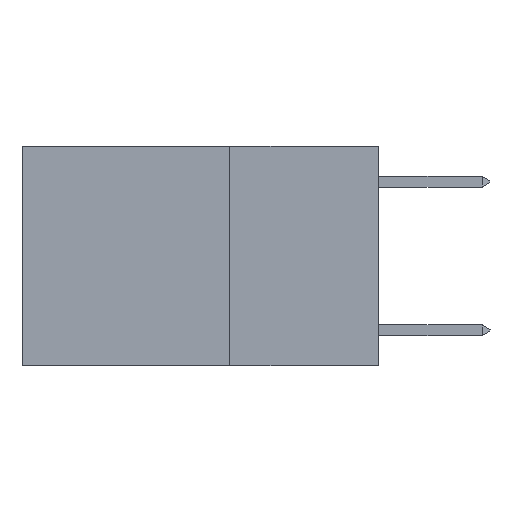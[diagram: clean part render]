
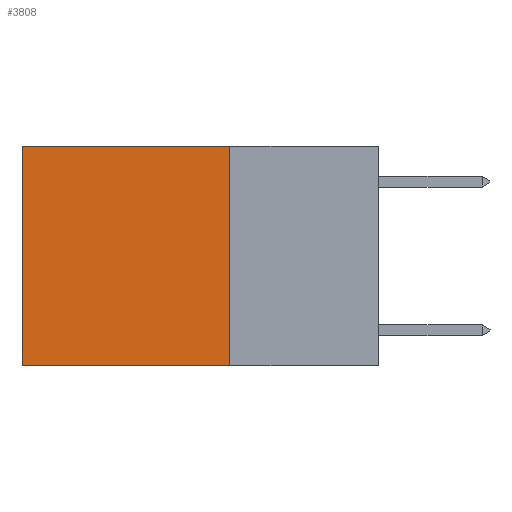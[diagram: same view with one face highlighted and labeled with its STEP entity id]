
A CAD part, left-side view. The second image highlights one B-rep face of the part: STEP entity #3808.
In plain terms, the highlighted planar face has unit normal (-1, 0, 0).
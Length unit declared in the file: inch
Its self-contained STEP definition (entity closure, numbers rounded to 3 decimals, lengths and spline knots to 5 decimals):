
#885 = CARTESIAN_POINT ( 'NONE',  ( 0.2625, 0.25, 0. ) ) ;
#1036 = VERTEX_POINT ( 'NONE', #885 ) ;
#1169 = CARTESIAN_POINT ( 'NONE',  ( 0.2625, 0.25, -0.37 ) ) ;
#1380 = DIRECTION ( 'NONE',  ( 0., 1., 0. ) ) ;
#1944 = VECTOR ( 'NONE', #23307, 39.37008 ) ;
#2574 = LINE ( 'NONE', #23353, #1944 ) ;
#2638 = EDGE_CURVE ( 'NONE', #3372, #15131, #9044, .T. ) ;
#2869 = EDGE_CURVE ( 'NONE', #1036, #23867, #6952, .T. ) ;
#3372 = VERTEX_POINT ( 'NONE', #23870 ) ;
#3589 = CARTESIAN_POINT ( 'NONE',  ( 0.2625, 0.6, -0.37 ) ) ;
#3808 = ADVANCED_FACE ( 'NONE', ( #20511 ), #8198, .F. ) ;
#4648 = ORIENTED_EDGE ( 'NONE', *, *, #2869, .F. ) ;
#4701 = ORIENTED_EDGE ( 'NONE', *, *, #2638, .T. ) ;
#6514 = VECTOR ( 'NONE', #7619, 39.37008 ) ;
#6952 = LINE ( 'NONE', #7565, #6514 ) ;
#7565 = CARTESIAN_POINT ( 'NONE',  ( 0.2625, 0.25, 0. ) ) ;
#7619 = DIRECTION ( 'NONE',  ( 0., 0., -1. ) ) ;
#7929 = DIRECTION ( 'NONE',  ( 0., 0., -1. ) ) ;
#7980 = DIRECTION ( 'NONE',  ( 1., 0., 0. ) ) ;
#8082 = CARTESIAN_POINT ( 'NONE',  ( 0.2625, 0.25, 0. ) ) ;
#8198 = PLANE ( 'NONE',  #23830 ) ;
#8759 = VECTOR ( 'NONE', #10515, 39.37008 ) ;
#8816 = ORIENTED_EDGE ( 'NONE', *, *, #11982, .F. ) ;
#9044 = LINE ( 'NONE', #10491, #8759 ) ;
#9880 = EDGE_CURVE ( 'NONE', #1036, #3372, #2574, .T. ) ;
#9975 = EDGE_LOOP ( 'NONE', ( #4701, #8816, #4648, #14585 ) ) ;
#10491 = CARTESIAN_POINT ( 'NONE',  ( 0.2625, 0.6, 0. ) ) ;
#10515 = DIRECTION ( 'NONE',  ( 0., 0., -1. ) ) ;
#11982 = EDGE_CURVE ( 'NONE', #23867, #15131, #12876, .T. ) ;
#12734 = VECTOR ( 'NONE', #1380, 39.37008 ) ;
#12876 = LINE ( 'NONE', #1169, #12734 ) ;
#14585 = ORIENTED_EDGE ( 'NONE', *, *, #9880, .T. ) ;
#15131 = VERTEX_POINT ( 'NONE', #3589 ) ;
#20511 = FACE_OUTER_BOUND ( 'NONE', #9975, .T. ) ;
#23307 = DIRECTION ( 'NONE',  ( 0., 1., 0. ) ) ;
#23353 = CARTESIAN_POINT ( 'NONE',  ( 0.2625, 0.25, 0. ) ) ;
#23707 = CARTESIAN_POINT ( 'NONE',  ( 0.2625, 0.25, -0.37 ) ) ;
#23830 = AXIS2_PLACEMENT_3D ( 'NONE', #8082, #7980, #7929 ) ;
#23867 = VERTEX_POINT ( 'NONE', #23707 ) ;
#23870 = CARTESIAN_POINT ( 'NONE',  ( 0.2625, 0.6, 0. ) ) ;
